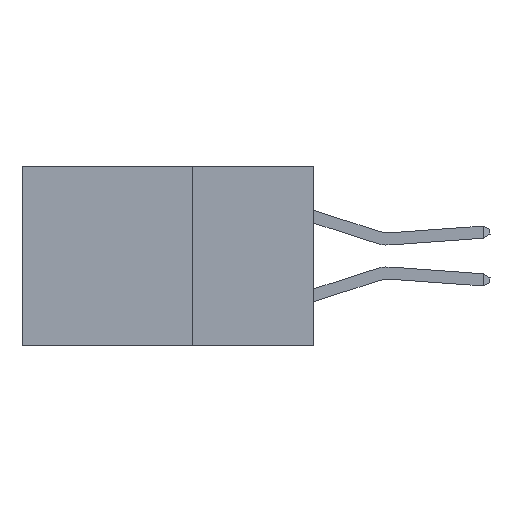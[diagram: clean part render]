
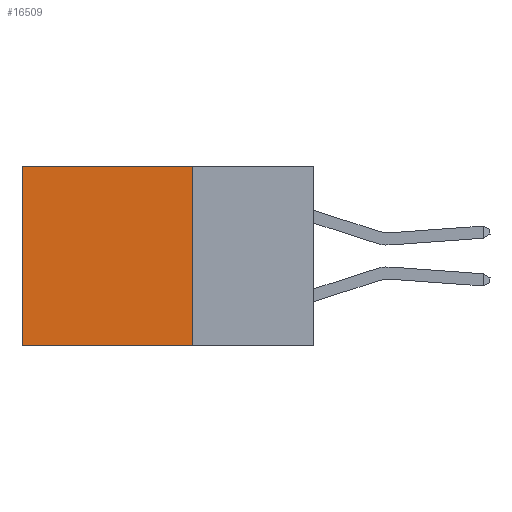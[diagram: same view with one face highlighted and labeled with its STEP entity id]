
A CAD part, left-side view. The second image highlights one B-rep face of the part: STEP entity #16509.
In plain terms, the highlighted planar face has unit normal (-1, 0, 0).
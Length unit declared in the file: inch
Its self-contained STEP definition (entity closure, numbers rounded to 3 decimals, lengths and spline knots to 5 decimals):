
#1137 = LINE ( 'NONE', #26276, #15045 ) ;
#2918 = EDGE_CURVE ( 'NONE', #32259, #16879, #10391, .T. ) ;
#3494 = PLANE ( 'NONE',  #20964 ) ;
#7688 = CARTESIAN_POINT ( 'NONE',  ( 0.2875, 0.25, 0. ) ) ;
#7771 = FACE_OUTER_BOUND ( 'NONE', #16913, .T. ) ;
#8979 = ORIENTED_EDGE ( 'NONE', *, *, #24684, .T. ) ;
#10391 = LINE ( 'NONE', #24479, #31355 ) ;
#10895 = DIRECTION ( 'NONE',  ( 0., 0., -1. ) ) ;
#11890 = CARTESIAN_POINT ( 'NONE',  ( 0.2875, 0.25, 0. ) ) ;
#13251 = DIRECTION ( 'NONE',  ( 0., 0., -1. ) ) ;
#13752 = CARTESIAN_POINT ( 'NONE',  ( 0.2875, 0.25, -0.37 ) ) ;
#13753 = EDGE_CURVE ( 'NONE', #25773, #16879, #22985, .T. ) ;
#14678 = DIRECTION ( 'NONE',  ( 0., 0., -1. ) ) ;
#14868 = CARTESIAN_POINT ( 'NONE',  ( 0.2875, 0.6, 0. ) ) ;
#15045 = VECTOR ( 'NONE', #29009, 39.37008 ) ;
#16509 = ADVANCED_FACE ( 'NONE', ( #7771 ), #3494, .F. ) ;
#16879 = VERTEX_POINT ( 'NONE', #18856 ) ;
#16913 = EDGE_LOOP ( 'NONE', ( #31874, #16923, #20694, #8979 ) ) ;
#16923 = ORIENTED_EDGE ( 'NONE', *, *, #2918, .F. ) ;
#18856 = CARTESIAN_POINT ( 'NONE',  ( 0.2875, 0.6, -0.37 ) ) ;
#20694 = ORIENTED_EDGE ( 'NONE', *, *, #23878, .F. ) ;
#20964 = AXIS2_PLACEMENT_3D ( 'NONE', #11890, #31017, #14678 ) ;
#22985 = LINE ( 'NONE', #30060, #30232 ) ;
#23878 = EDGE_CURVE ( 'NONE', #30579, #32259, #33446, .T. ) ;
#24051 = CARTESIAN_POINT ( 'NONE',  ( 0.2875, 0.25, 0. ) ) ;
#24479 = CARTESIAN_POINT ( 'NONE',  ( 0.2875, 0.25, -0.37 ) ) ;
#24684 = EDGE_CURVE ( 'NONE', #30579, #25773, #1137, .T. ) ;
#25773 = VERTEX_POINT ( 'NONE', #14868 ) ;
#26227 = VECTOR ( 'NONE', #13251, 39.37008 ) ;
#26276 = CARTESIAN_POINT ( 'NONE',  ( 0.2875, 0.25, 0. ) ) ;
#27202 = DIRECTION ( 'NONE',  ( 0., 1., 0. ) ) ;
#29009 = DIRECTION ( 'NONE',  ( 0., 1., 0. ) ) ;
#30060 = CARTESIAN_POINT ( 'NONE',  ( 0.2875, 0.6, 0. ) ) ;
#30232 = VECTOR ( 'NONE', #10895, 39.37008 ) ;
#30579 = VERTEX_POINT ( 'NONE', #24051 ) ;
#31017 = DIRECTION ( 'NONE',  ( 1., 0., 0. ) ) ;
#31355 = VECTOR ( 'NONE', #27202, 39.37008 ) ;
#31874 = ORIENTED_EDGE ( 'NONE', *, *, #13753, .T. ) ;
#32259 = VERTEX_POINT ( 'NONE', #13752 ) ;
#33446 = LINE ( 'NONE', #7688, #26227 ) ;
